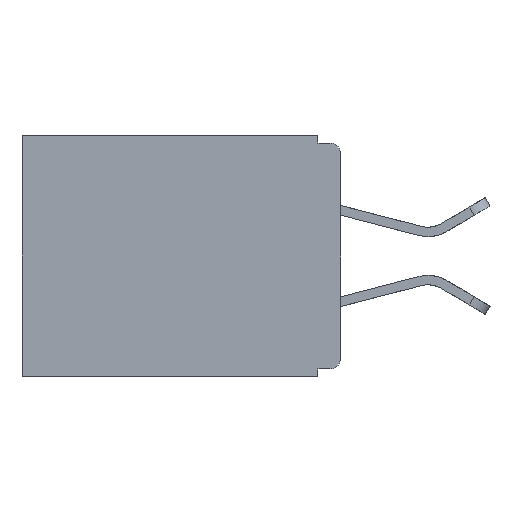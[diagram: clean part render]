
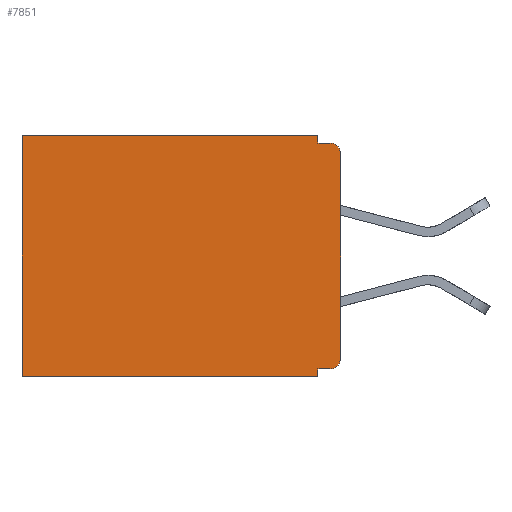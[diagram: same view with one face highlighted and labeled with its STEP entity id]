
A CAD part, left-side view. The second image highlights one B-rep face of the part: STEP entity #7851.
In plain terms, the highlighted planar face has unit normal (-1, 0, 0).
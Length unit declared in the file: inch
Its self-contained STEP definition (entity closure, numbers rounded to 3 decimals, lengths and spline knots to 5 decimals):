
#41 = ORIENTED_EDGE ( 'NONE', *, *, #11297, .F. ) ;
#228 = EDGE_LOOP ( 'NONE', ( #41, #17834, #24314, #4241, #27093, #11047, #6593, #5500, #20104, #11410 ) ) ;
#835 = VERTEX_POINT ( 'NONE', #15698 ) ;
#2255 = CARTESIAN_POINT ( 'NONE',  ( 0.3, 0.031, 0. ) ) ;
#2441 = AXIS2_PLACEMENT_3D ( 'NONE', #24176, #9007, #26617 ) ;
#2869 = CARTESIAN_POINT ( 'NONE',  ( 0.3, 0.031, -0.32 ) ) ;
#3149 = CARTESIAN_POINT ( 'NONE',  ( 0.3, 0.031, -0.33 ) ) ;
#3903 = DIRECTION ( 'NONE',  ( 0., -1., 0. ) ) ;
#4056 = EDGE_CURVE ( 'NONE', #15579, #14499, #4237, .T. ) ;
#4237 = LINE ( 'NONE', #11564, #17111 ) ;
#4241 = ORIENTED_EDGE ( 'NONE', *, *, #12241, .F. ) ;
#4655 = DIRECTION ( 'NONE',  ( 0., 0., -1. ) ) ;
#4849 = CARTESIAN_POINT ( 'NONE',  ( 0.3, 0.031, 0. ) ) ;
#5500 = ORIENTED_EDGE ( 'NONE', *, *, #23157, .F. ) ;
#5828 = CARTESIAN_POINT ( 'NONE',  ( 0.3, 0.031, -0.01 ) ) ;
#6073 = LINE ( 'NONE', #15808, #19726 ) ;
#6347 = VERTEX_POINT ( 'NONE', #2869 ) ;
#6593 = ORIENTED_EDGE ( 'NONE', *, *, #30417, .F. ) ;
#7115 = VERTEX_POINT ( 'NONE', #25765 ) ;
#7851 = ADVANCED_FACE ( 'NONE', ( #25867 ), #15936, .F. ) ;
#9007 = DIRECTION ( 'NONE',  ( -1., 0., 0. ) ) ;
#9601 = CARTESIAN_POINT ( 'NONE',  ( 0.3, 0., -0.305 ) ) ;
#9678 = LINE ( 'NONE', #18981, #15687 ) ;
#11047 = ORIENTED_EDGE ( 'NONE', *, *, #4056, .T. ) ;
#11242 = EDGE_CURVE ( 'NONE', #20099, #13525, #28095, .T. ) ;
#11297 = EDGE_CURVE ( 'NONE', #7115, #13525, #19992, .T. ) ;
#11410 = ORIENTED_EDGE ( 'NONE', *, *, #11242, .T. ) ;
#11564 = CARTESIAN_POINT ( 'NONE',  ( 0.3, 0.437, -0.33 ) ) ;
#12241 = EDGE_CURVE ( 'NONE', #19526, #28123, #19936, .T. ) ;
#13042 = CIRCLE ( 'NONE', #2441, 0.015 ) ;
#13525 = VERTEX_POINT ( 'NONE', #9601 ) ;
#13536 = VECTOR ( 'NONE', #3903, 39.37008 ) ;
#14499 = VERTEX_POINT ( 'NONE', #26334 ) ;
#14638 = VECTOR ( 'NONE', #25294, 39.37008 ) ;
#15579 = VERTEX_POINT ( 'NONE', #30308 ) ;
#15687 = VECTOR ( 'NONE', #31305, 39.37008 ) ;
#15698 = CARTESIAN_POINT ( 'NONE',  ( 0.3, 0.015, -0.01 ) ) ;
#15739 = DIRECTION ( 'NONE',  ( 0., 0., -1. ) ) ;
#15790 = DIRECTION ( 'NONE',  ( 1., 0., 0. ) ) ;
#15808 = CARTESIAN_POINT ( 'NONE',  ( 0.3, 0., -0.33 ) ) ;
#15898 = CARTESIAN_POINT ( 'NONE',  ( 0.3, 0., -0.33 ) ) ;
#15936 = PLANE ( 'NONE',  #24874 ) ;
#16257 = LINE ( 'NONE', #32492, #14638 ) ;
#16632 = LINE ( 'NONE', #30642, #22526 ) ;
#16731 = CARTESIAN_POINT ( 'NONE',  ( 0.3, 0., -0.01 ) ) ;
#17111 = VECTOR ( 'NONE', #22975, 39.37008 ) ;
#17834 = ORIENTED_EDGE ( 'NONE', *, *, #27661, .T. ) ;
#17911 = VERTEX_POINT ( 'NONE', #3149 ) ;
#18029 = EDGE_CURVE ( 'NONE', #20099, #6347, #9678, .T. ) ;
#18981 = CARTESIAN_POINT ( 'NONE',  ( 0.3, 0., -0.32 ) ) ;
#19526 = VERTEX_POINT ( 'NONE', #2255 ) ;
#19726 = VECTOR ( 'NONE', #30637, 39.37008 ) ;
#19936 = LINE ( 'NONE', #4849, #24954 ) ;
#19992 = LINE ( 'NONE', #25446, #25801 ) ;
#20099 = VERTEX_POINT ( 'NONE', #22067 ) ;
#20104 = ORIENTED_EDGE ( 'NONE', *, *, #18029, .F. ) ;
#20359 = LINE ( 'NONE', #16731, #13536 ) ;
#20903 = DIRECTION ( 'NONE',  ( 0., 1., 0. ) ) ;
#21065 = AXIS2_PLACEMENT_3D ( 'NONE', #26286, #26154, #26143 ) ;
#21172 = EDGE_CURVE ( 'NONE', #28123, #835, #20359, .T. ) ;
#22067 = CARTESIAN_POINT ( 'NONE',  ( 0.3, 0.015, -0.32 ) ) ;
#22526 = VECTOR ( 'NONE', #20903, 39.37008 ) ;
#22975 = DIRECTION ( 'NONE',  ( 0., 0., -1. ) ) ;
#23157 = EDGE_CURVE ( 'NONE', #6347, #17911, #16257, .T. ) ;
#24176 = CARTESIAN_POINT ( 'NONE',  ( 0.3, 0.015, -0.025 ) ) ;
#24314 = ORIENTED_EDGE ( 'NONE', *, *, #21172, .F. ) ;
#24874 = AXIS2_PLACEMENT_3D ( 'NONE', #15898, #15790, #15739 ) ;
#24954 = VECTOR ( 'NONE', #4655, 39.37008 ) ;
#25294 = DIRECTION ( 'NONE',  ( 0., 0., -1. ) ) ;
#25378 = DIRECTION ( 'NONE',  ( 0., 0., -1. ) ) ;
#25446 = CARTESIAN_POINT ( 'NONE',  ( 0.3, 0., -0.33 ) ) ;
#25765 = CARTESIAN_POINT ( 'NONE',  ( 0.3, 0., -0.025 ) ) ;
#25801 = VECTOR ( 'NONE', #25378, 39.37008 ) ;
#25867 = FACE_OUTER_BOUND ( 'NONE', #228, .T. ) ;
#26143 = DIRECTION ( 'NONE',  ( 0., 0., -1. ) ) ;
#26154 = DIRECTION ( 'NONE',  ( -1., 0., 0. ) ) ;
#26286 = CARTESIAN_POINT ( 'NONE',  ( 0.3, 0.015, -0.305 ) ) ;
#26334 = CARTESIAN_POINT ( 'NONE',  ( 0.3, 0.437, -0.33 ) ) ;
#26617 = DIRECTION ( 'NONE',  ( 0., 0., -1. ) ) ;
#27093 = ORIENTED_EDGE ( 'NONE', *, *, #28589, .T. ) ;
#27661 = EDGE_CURVE ( 'NONE', #7115, #835, #13042, .T. ) ;
#28095 = CIRCLE ( 'NONE', #21065, 0.015 ) ;
#28123 = VERTEX_POINT ( 'NONE', #5828 ) ;
#28589 = EDGE_CURVE ( 'NONE', #19526, #15579, #16632, .T. ) ;
#30308 = CARTESIAN_POINT ( 'NONE',  ( 0.3, 0.437, 0. ) ) ;
#30417 = EDGE_CURVE ( 'NONE', #17911, #14499, #6073, .T. ) ;
#30637 = DIRECTION ( 'NONE',  ( 0., 1., 0. ) ) ;
#30642 = CARTESIAN_POINT ( 'NONE',  ( 0.3, 0., 0. ) ) ;
#31305 = DIRECTION ( 'NONE',  ( 0., 1., 0. ) ) ;
#32492 = CARTESIAN_POINT ( 'NONE',  ( 0.3, 0.031, -0.33 ) ) ;
